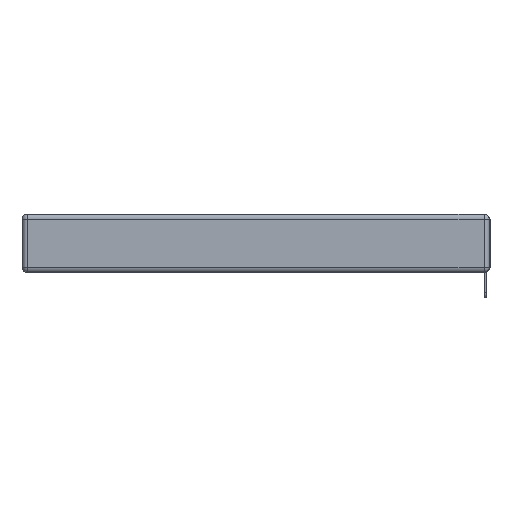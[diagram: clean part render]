
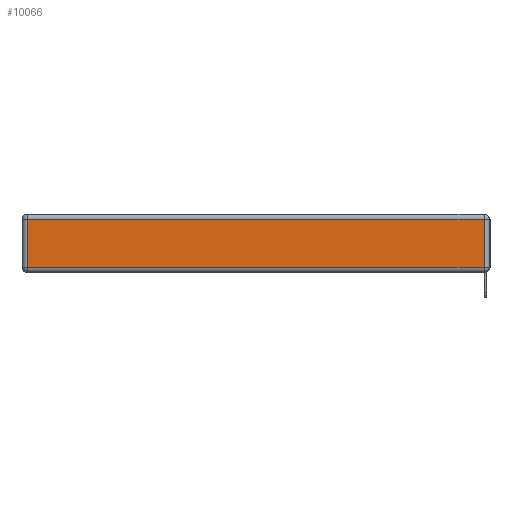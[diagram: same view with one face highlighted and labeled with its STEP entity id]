
A CAD part, left-side view. The second image highlights one B-rep face of the part: STEP entity #10066.
In plain terms, the highlighted planar face has unit normal (-1, 0, 0).
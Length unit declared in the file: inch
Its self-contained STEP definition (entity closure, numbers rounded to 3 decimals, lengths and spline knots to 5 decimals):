
#143 = LINE ( 'NONE', #3856, #3672 ) ;
#1473 = LINE ( 'NONE', #19293, #18363 ) ;
#1905 = EDGE_CURVE ( 'NONE', #20985, #15172, #9677, .T. ) ;
#2335 = CARTESIAN_POINT ( 'NONE',  ( 0., 2.72, -0.313 ) ) ;
#3672 = VECTOR ( 'NONE', #9277, 39.37008 ) ;
#3856 = CARTESIAN_POINT ( 'NONE',  ( 0., 0., -0.313 ) ) ;
#4997 = CARTESIAN_POINT ( 'NONE',  ( 0., 0., -0.343 ) ) ;
#6309 = EDGE_LOOP ( 'NONE', ( #18362, #11335, #19177, #8297 ) ) ;
#6764 = EDGE_CURVE ( 'NONE', #15172, #17622, #7235, .T. ) ;
#6783 = DIRECTION ( 'NONE',  ( 0., 0., -1. ) ) ;
#6958 = DIRECTION ( 'NONE',  ( 0., 0., 1. ) ) ;
#7235 = LINE ( 'NONE', #21134, #9284 ) ;
#8297 = ORIENTED_EDGE ( 'NONE', *, *, #6764, .T. ) ;
#8578 = DIRECTION ( 'NONE',  ( -1., 0., 0. ) ) ;
#9277 = DIRECTION ( 'NONE',  ( 0., -1., 0. ) ) ;
#9284 = VECTOR ( 'NONE', #6783, 39.37008 ) ;
#9451 = CARTESIAN_POINT ( 'NONE',  ( 0., 2.75, -0.03 ) ) ;
#9677 = LINE ( 'NONE', #9451, #17393 ) ;
#10066 = ADVANCED_FACE ( 'NONE', ( #19005 ), #22809, .T. ) ;
#10476 = DIRECTION ( 'NONE',  ( 0., 0., 1. ) ) ;
#11335 = ORIENTED_EDGE ( 'NONE', *, *, #13108, .T. ) ;
#13108 = EDGE_CURVE ( 'NONE', #13172, #20985, #1473, .T. ) ;
#13172 = VERTEX_POINT ( 'NONE', #14523 ) ;
#14027 = CARTESIAN_POINT ( 'NONE',  ( 0., 2.72, -0.03 ) ) ;
#14523 = CARTESIAN_POINT ( 'NONE',  ( 0., 0.03, -0.313 ) ) ;
#15172 = VERTEX_POINT ( 'NONE', #14027 ) ;
#16636 = DIRECTION ( 'NONE',  ( 0., 1., 0. ) ) ;
#16764 = AXIS2_PLACEMENT_3D ( 'NONE', #4997, #8578, #6958 ) ;
#17393 = VECTOR ( 'NONE', #16636, 39.37008 ) ;
#17622 = VERTEX_POINT ( 'NONE', #2335 ) ;
#18362 = ORIENTED_EDGE ( 'NONE', *, *, #22772, .T. ) ;
#18363 = VECTOR ( 'NONE', #10476, 39.37008 ) ;
#19005 = FACE_OUTER_BOUND ( 'NONE', #6309, .T. ) ;
#19177 = ORIENTED_EDGE ( 'NONE', *, *, #1905, .T. ) ;
#19293 = CARTESIAN_POINT ( 'NONE',  ( 0., 0.03, -0.343 ) ) ;
#20985 = VERTEX_POINT ( 'NONE', #21350 ) ;
#21134 = CARTESIAN_POINT ( 'NONE',  ( 0., 2.72, -0.343 ) ) ;
#21350 = CARTESIAN_POINT ( 'NONE',  ( 0., 0.03, -0.03 ) ) ;
#22772 = EDGE_CURVE ( 'NONE', #17622, #13172, #143, .T. ) ;
#22809 = PLANE ( 'NONE',  #16764 ) ;
